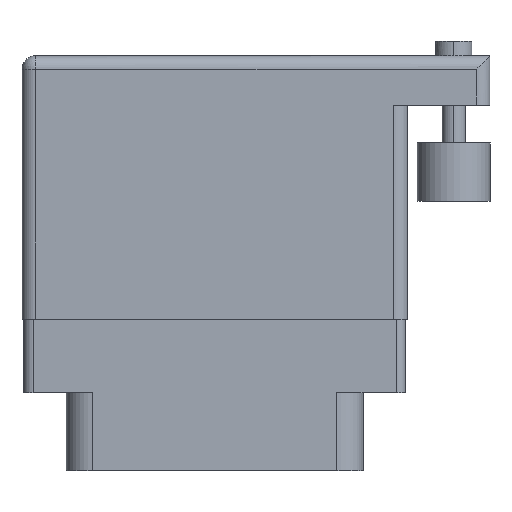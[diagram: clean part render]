
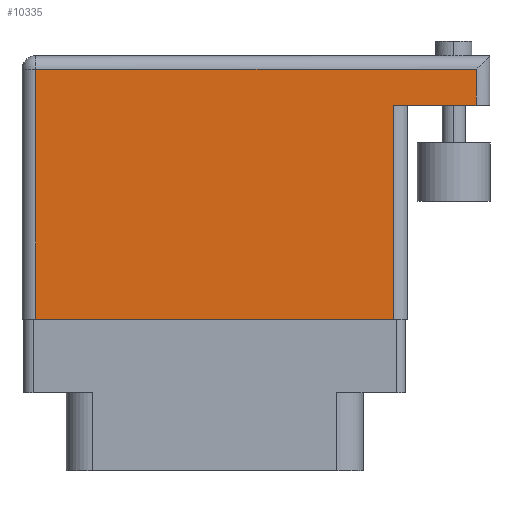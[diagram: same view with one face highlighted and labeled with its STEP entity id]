
A CAD part, front view. The second image highlights one B-rep face of the part: STEP entity #10335.
In plain terms, the highlighted face is planar.
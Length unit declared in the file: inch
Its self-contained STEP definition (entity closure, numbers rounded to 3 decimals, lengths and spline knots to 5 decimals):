
#946 = DIRECTION ( 'NONE',  ( -1., 0., 0. ) ) ;
#1564 = CARTESIAN_POINT ( 'NONE',  ( 0., 0.906, 0. ) ) ;
#1671 = EDGE_CURVE ( 'NONE', #17918, #15699, #2200, .T. ) ;
#2200 = LINE ( 'NONE', #8754, #3778 ) ;
#2333 = ORIENTED_EDGE ( 'NONE', *, *, #18195, .F. ) ;
#2592 = ORIENTED_EDGE ( 'NONE', *, *, #19422, .T. ) ;
#2710 = ORIENTED_EDGE ( 'NONE', *, *, #15550, .T. ) ;
#3778 = VECTOR ( 'NONE', #8980, 39.37008 ) ;
#3829 = LINE ( 'NONE', #7058, #14527 ) ;
#5203 = EDGE_CURVE ( 'NONE', #6563, #17918, #3829, .T. ) ;
#5351 = LINE ( 'NONE', #12108, #21146 ) ;
#6025 = DIRECTION ( 'NONE',  ( 0., 1., 0. ) ) ;
#6563 = VERTEX_POINT ( 'NONE', #10294 ) ;
#7058 = CARTESIAN_POINT ( 'NONE',  ( 0., 0., 0. ) ) ;
#7606 = LINE ( 'NONE', #14357, #15087 ) ;
#7879 = EDGE_LOOP ( 'NONE', ( #15741, #13283, #2333, #13705, #2592, #2710 ) ) ;
#8097 = VERTEX_POINT ( 'NONE', #15083 ) ;
#8271 = CARTESIAN_POINT ( 'NONE',  ( 1.278, 0., 0. ) ) ;
#8301 = CARTESIAN_POINT ( 'NONE',  ( 0.047, 0., 0. ) ) ;
#8754 = CARTESIAN_POINT ( 'NONE',  ( 1.278, 0.736, 0. ) ) ;
#8980 = DIRECTION ( 'NONE',  ( 0., 1., 0. ) ) ;
#10294 = CARTESIAN_POINT ( 'NONE',  ( 0.047, 0., 0. ) ) ;
#10335 = ADVANCED_FACE ( 'NONE', ( #16750 ), #16650, .F. ) ;
#11887 = DIRECTION ( 'NONE',  ( -1., 0., 0. ) ) ;
#12108 = CARTESIAN_POINT ( 'NONE',  ( 0., 0.859, 0. ) ) ;
#12515 = AXIS2_PLACEMENT_3D ( 'NONE', #1564, #21826, #13429 ) ;
#13283 = ORIENTED_EDGE ( 'NONE', *, *, #1671, .T. ) ;
#13429 = DIRECTION ( 'NONE',  ( -1., 0., 0. ) ) ;
#13705 = ORIENTED_EDGE ( 'NONE', *, *, #19717, .T. ) ;
#13809 = DIRECTION ( 'NONE',  ( 1., 0., 0. ) ) ;
#14357 = CARTESIAN_POINT ( 'NONE',  ( 1.609, 0.736, 0. ) ) ;
#14527 = VECTOR ( 'NONE', #13809, 39.37008 ) ;
#15054 = DIRECTION ( 'NONE',  ( 0., -1., 0. ) ) ;
#15083 = CARTESIAN_POINT ( 'NONE',  ( 0.047, 0.859, 0. ) ) ;
#15087 = VECTOR ( 'NONE', #946, 39.37008 ) ;
#15550 = EDGE_CURVE ( 'NONE', #8097, #6563, #21789, .T. ) ;
#15699 = VERTEX_POINT ( 'NONE', #17696 ) ;
#15741 = ORIENTED_EDGE ( 'NONE', *, *, #5203, .T. ) ;
#16253 = CARTESIAN_POINT ( 'NONE',  ( 1.562, 0.736, 0. ) ) ;
#16488 = CARTESIAN_POINT ( 'NONE',  ( 1.562, 0.859, 0. ) ) ;
#16521 = LINE ( 'NONE', #21295, #17952 ) ;
#16650 = PLANE ( 'NONE',  #12515 ) ;
#16750 = FACE_OUTER_BOUND ( 'NONE', #7879, .T. ) ;
#17696 = CARTESIAN_POINT ( 'NONE',  ( 1.278, 0.736, 0. ) ) ;
#17918 = VERTEX_POINT ( 'NONE', #8271 ) ;
#17952 = VECTOR ( 'NONE', #6025, 39.37008 ) ;
#18195 = EDGE_CURVE ( 'NONE', #21690, #15699, #7606, .T. ) ;
#19422 = EDGE_CURVE ( 'NONE', #21205, #8097, #5351, .T. ) ;
#19717 = EDGE_CURVE ( 'NONE', #21690, #21205, #16521, .T. ) ;
#20540 = VECTOR ( 'NONE', #15054, 39.37008 ) ;
#21146 = VECTOR ( 'NONE', #11887, 39.37008 ) ;
#21205 = VERTEX_POINT ( 'NONE', #16488 ) ;
#21295 = CARTESIAN_POINT ( 'NONE',  ( 1.562, 0.906, 0. ) ) ;
#21690 = VERTEX_POINT ( 'NONE', #16253 ) ;
#21789 = LINE ( 'NONE', #8301, #20540 ) ;
#21826 = DIRECTION ( 'NONE',  ( 0., 0., -1. ) ) ;
